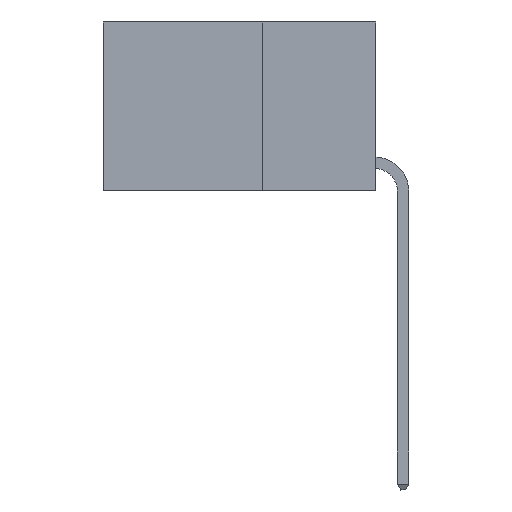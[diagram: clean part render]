
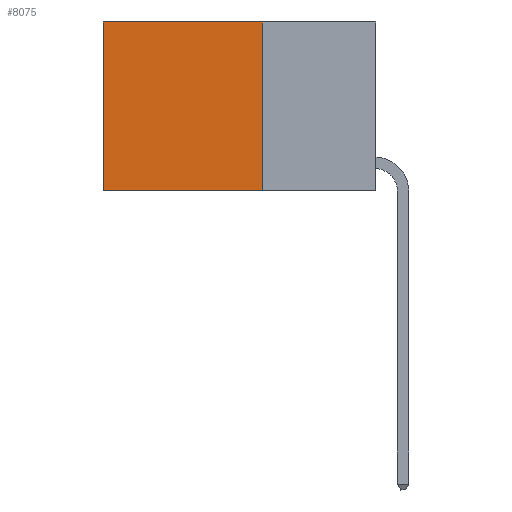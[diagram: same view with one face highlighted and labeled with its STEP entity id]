
A CAD part, left-side view. The second image highlights one B-rep face of the part: STEP entity #8075.
In plain terms, the highlighted planar face has unit normal (-1, 0, 0).
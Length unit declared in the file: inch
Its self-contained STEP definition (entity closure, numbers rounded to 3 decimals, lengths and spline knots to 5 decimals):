
#611 = EDGE_CURVE ( 'NONE', #8946, #2196, #16388, .T. ) ;
#2196 = VERTEX_POINT ( 'NONE', #11135 ) ;
#2292 = CARTESIAN_POINT ( 'NONE',  ( 0.2625, 0.25, 0. ) ) ;
#2462 = CARTESIAN_POINT ( 'NONE',  ( 0.2625, 0.6, -0.37 ) ) ;
#3767 = LINE ( 'NONE', #25077, #5570 ) ;
#4787 = CARTESIAN_POINT ( 'NONE',  ( 0.2625, 0.25, 0. ) ) ;
#5115 = LINE ( 'NONE', #16703, #27622 ) ;
#5570 = VECTOR ( 'NONE', #17827, 39.37008 ) ;
#6287 = CARTESIAN_POINT ( 'NONE',  ( 0.2625, 0.25, 0. ) ) ;
#8075 = ADVANCED_FACE ( 'NONE', ( #15260 ), #27276, .F. ) ;
#8244 = LINE ( 'NONE', #24757, #19225 ) ;
#8946 = VERTEX_POINT ( 'NONE', #2292 ) ;
#9190 = CARTESIAN_POINT ( 'NONE',  ( 0.2625, 0.25, -0.37 ) ) ;
#11135 = CARTESIAN_POINT ( 'NONE',  ( 0.2625, 0.6, 0. ) ) ;
#13162 = ORIENTED_EDGE ( 'NONE', *, *, #21266, .F. ) ;
#14202 = ORIENTED_EDGE ( 'NONE', *, *, #16359, .T. ) ;
#14402 = DIRECTION ( 'NONE',  ( 0., 0., -1. ) ) ;
#14523 = DIRECTION ( 'NONE',  ( 0., 1., 0. ) ) ;
#14649 = AXIS2_PLACEMENT_3D ( 'NONE', #6287, #18021, #22498 ) ;
#15260 = FACE_OUTER_BOUND ( 'NONE', #19712, .T. ) ;
#15860 = ORIENTED_EDGE ( 'NONE', *, *, #611, .T. ) ;
#16359 = EDGE_CURVE ( 'NONE', #2196, #21718, #3767, .T. ) ;
#16388 = LINE ( 'NONE', #4787, #21838 ) ;
#16703 = CARTESIAN_POINT ( 'NONE',  ( 0.2625, 0.25, 0. ) ) ;
#17827 = DIRECTION ( 'NONE',  ( 0., 0., -1. ) ) ;
#18021 = DIRECTION ( 'NONE',  ( 1., 0., 0. ) ) ;
#19101 = VERTEX_POINT ( 'NONE', #9190 ) ;
#19225 = VECTOR ( 'NONE', #27225, 39.37008 ) ;
#19712 = EDGE_LOOP ( 'NONE', ( #14202, #20906, #13162, #15860 ) ) ;
#20906 = ORIENTED_EDGE ( 'NONE', *, *, #20961, .F. ) ;
#20961 = EDGE_CURVE ( 'NONE', #19101, #21718, #8244, .T. ) ;
#21266 = EDGE_CURVE ( 'NONE', #8946, #19101, #5115, .T. ) ;
#21718 = VERTEX_POINT ( 'NONE', #2462 ) ;
#21838 = VECTOR ( 'NONE', #14523, 39.37008 ) ;
#22498 = DIRECTION ( 'NONE',  ( 0., 0., -1. ) ) ;
#24757 = CARTESIAN_POINT ( 'NONE',  ( 0.2625, 0.25, -0.37 ) ) ;
#25077 = CARTESIAN_POINT ( 'NONE',  ( 0.2625, 0.6, 0. ) ) ;
#27225 = DIRECTION ( 'NONE',  ( 0., 1., 0. ) ) ;
#27276 = PLANE ( 'NONE',  #14649 ) ;
#27622 = VECTOR ( 'NONE', #14402, 39.37008 ) ;
